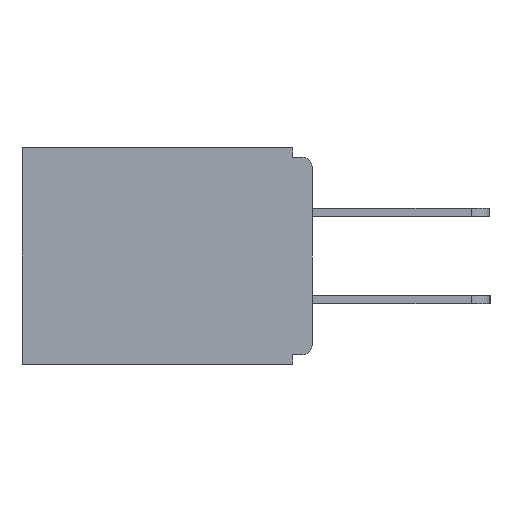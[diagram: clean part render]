
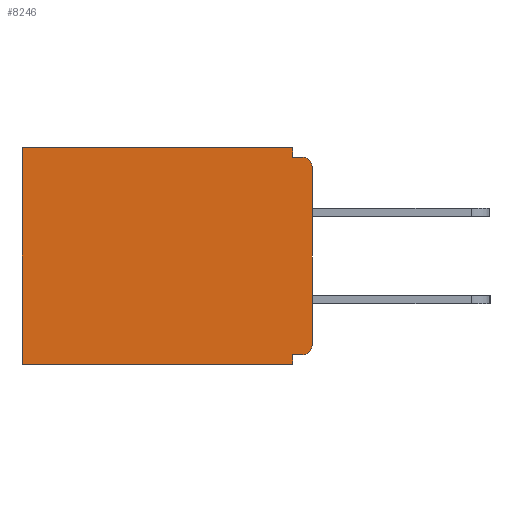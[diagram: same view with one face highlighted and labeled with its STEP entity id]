
A CAD part, left-side view. The second image highlights one B-rep face of the part: STEP entity #8246.
In plain terms, the highlighted planar face has unit normal (-1, 0, 0).
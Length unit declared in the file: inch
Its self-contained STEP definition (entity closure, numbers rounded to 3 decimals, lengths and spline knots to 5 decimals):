
#279 = VECTOR ( 'NONE', #2472, 39.37008 ) ;
#393 = VERTEX_POINT ( 'NONE', #2264 ) ;
#464 = CARTESIAN_POINT ( 'NONE',  ( 0.298, 0.031, -0.343 ) ) ;
#641 = DIRECTION ( 'NONE',  ( 0., 0., -1. ) ) ;
#651 = VERTEX_POINT ( 'NONE', #9952 ) ;
#726 = CARTESIAN_POINT ( 'NONE',  ( 0.298, 0., -0.328 ) ) ;
#794 = VERTEX_POINT ( 'NONE', #1042 ) ;
#1023 = LINE ( 'NONE', #1799, #2054 ) ;
#1042 = CARTESIAN_POINT ( 'NONE',  ( 0.298, 0.015, -0.328 ) ) ;
#1272 = VECTOR ( 'NONE', #8015, 39.37008 ) ;
#1454 = ORIENTED_EDGE ( 'NONE', *, *, #10902, .T. ) ;
#1741 = EDGE_CURVE ( 'NONE', #5971, #651, #8918, .T. ) ;
#1799 = CARTESIAN_POINT ( 'NONE',  ( 0.298, 0., -0.015 ) ) ;
#1800 = CIRCLE ( 'NONE', #10659, 0.015 ) ;
#1918 = ORIENTED_EDGE ( 'NONE', *, *, #3690, .F. ) ;
#2054 = VECTOR ( 'NONE', #12324, 39.37008 ) ;
#2264 = CARTESIAN_POINT ( 'NONE',  ( 0.298, 0.031, -0.015 ) ) ;
#2284 = LINE ( 'NONE', #4852, #12710 ) ;
#2448 = ORIENTED_EDGE ( 'NONE', *, *, #1741, .F. ) ;
#2472 = DIRECTION ( 'NONE',  ( 0., 0., -1. ) ) ;
#2620 = DIRECTION ( 'NONE',  ( -1., 0., 0. ) ) ;
#2828 = PLANE ( 'NONE',  #9819 ) ;
#3073 = VERTEX_POINT ( 'NONE', #3574 ) ;
#3208 = ORIENTED_EDGE ( 'NONE', *, *, #4768, .T. ) ;
#3418 = ORIENTED_EDGE ( 'NONE', *, *, #12832, .T. ) ;
#3472 = CARTESIAN_POINT ( 'NONE',  ( 0.298, 0., 0. ) ) ;
#3574 = CARTESIAN_POINT ( 'NONE',  ( 0.298, 0.031, 0. ) ) ;
#3594 = FACE_OUTER_BOUND ( 'NONE', #8398, .T. ) ;
#3690 = EDGE_CURVE ( 'NONE', #794, #4728, #9856, .T. ) ;
#3745 = VERTEX_POINT ( 'NONE', #13496 ) ;
#3828 = CARTESIAN_POINT ( 'NONE',  ( 0.298, 0.031, -0.328 ) ) ;
#4167 = DIRECTION ( 'NONE',  ( -1., 0., 0. ) ) ;
#4298 = CARTESIAN_POINT ( 'NONE',  ( 0.298, 0.015, -0.313 ) ) ;
#4319 = VECTOR ( 'NONE', #5963, 39.37008 ) ;
#4413 = DIRECTION ( 'NONE',  ( 0., 0., -1. ) ) ;
#4554 = DIRECTION ( 'NONE',  ( 0., 1., 0. ) ) ;
#4728 = VERTEX_POINT ( 'NONE', #3828 ) ;
#4768 = EDGE_CURVE ( 'NONE', #5971, #13236, #5404, .T. ) ;
#4852 = CARTESIAN_POINT ( 'NONE',  ( 0.298, 0., -0.343 ) ) ;
#4991 = LINE ( 'NONE', #464, #279 ) ;
#5404 = CIRCLE ( 'NONE', #7848, 0.015 ) ;
#5413 = EDGE_CURVE ( 'NONE', #794, #651, #1800, .T. ) ;
#5963 = DIRECTION ( 'NONE',  ( 0., 1., 0. ) ) ;
#5968 = EDGE_CURVE ( 'NONE', #8989, #3745, #2284, .T. ) ;
#5971 = VERTEX_POINT ( 'NONE', #11239 ) ;
#6232 = VECTOR ( 'NONE', #4554, 39.37008 ) ;
#6331 = VECTOR ( 'NONE', #9665, 39.37008 ) ;
#6560 = ORIENTED_EDGE ( 'NONE', *, *, #7855, .F. ) ;
#6593 = VECTOR ( 'NONE', #4413, 39.37008 ) ;
#6707 = LINE ( 'NONE', #3472, #6232 ) ;
#6927 = CARTESIAN_POINT ( 'NONE',  ( 0.298, 0., 0. ) ) ;
#7169 = CARTESIAN_POINT ( 'NONE',  ( 0.298, 0.031, -0.343 ) ) ;
#7713 = VERTEX_POINT ( 'NONE', #8289 ) ;
#7799 = LINE ( 'NONE', #11717, #6331 ) ;
#7848 = AXIS2_PLACEMENT_3D ( 'NONE', #11018, #2620, #10045 ) ;
#7855 = EDGE_CURVE ( 'NONE', #3073, #393, #7799, .T. ) ;
#7961 = EDGE_CURVE ( 'NONE', #393, #13236, #1023, .T. ) ;
#8015 = DIRECTION ( 'NONE',  ( 0., 0., -1. ) ) ;
#8246 = ADVANCED_FACE ( 'NONE', ( #3594 ), #2828, .F. ) ;
#8289 = CARTESIAN_POINT ( 'NONE',  ( 0.298, 0.46, 0. ) ) ;
#8398 = EDGE_LOOP ( 'NONE', ( #3208, #10143, #6560, #3418, #1454, #13165, #8598, #1918, #12893, #2448 ) ) ;
#8598 = ORIENTED_EDGE ( 'NONE', *, *, #9366, .F. ) ;
#8918 = LINE ( 'NONE', #6927, #1272 ) ;
#8989 = VERTEX_POINT ( 'NONE', #7169 ) ;
#9366 = EDGE_CURVE ( 'NONE', #4728, #8989, #4991, .T. ) ;
#9665 = DIRECTION ( 'NONE',  ( 0., 0., -1. ) ) ;
#9819 = AXIS2_PLACEMENT_3D ( 'NONE', #13175, #10062, #641 ) ;
#9856 = LINE ( 'NONE', #726, #4319 ) ;
#9952 = CARTESIAN_POINT ( 'NONE',  ( 0.298, 0., -0.313 ) ) ;
#10045 = DIRECTION ( 'NONE',  ( 0., 0., -1. ) ) ;
#10062 = DIRECTION ( 'NONE',  ( 1., 0., 0. ) ) ;
#10081 = DIRECTION ( 'NONE',  ( 0., 1., 0. ) ) ;
#10143 = ORIENTED_EDGE ( 'NONE', *, *, #7961, .F. ) ;
#10659 = AXIS2_PLACEMENT_3D ( 'NONE', #4298, #4167, #13509 ) ;
#10706 = CARTESIAN_POINT ( 'NONE',  ( 0.298, 0.46, 0. ) ) ;
#10902 = EDGE_CURVE ( 'NONE', #7713, #3745, #12144, .T. ) ;
#11018 = CARTESIAN_POINT ( 'NONE',  ( 0.298, 0.015, -0.03 ) ) ;
#11239 = CARTESIAN_POINT ( 'NONE',  ( 0.298, 0., -0.03 ) ) ;
#11717 = CARTESIAN_POINT ( 'NONE',  ( 0.298, 0.031, -0.343 ) ) ;
#12144 = LINE ( 'NONE', #10706, #6593 ) ;
#12324 = DIRECTION ( 'NONE',  ( 0., -1., 0. ) ) ;
#12637 = CARTESIAN_POINT ( 'NONE',  ( 0.298, 0.015, -0.015 ) ) ;
#12710 = VECTOR ( 'NONE', #10081, 39.37008 ) ;
#12832 = EDGE_CURVE ( 'NONE', #3073, #7713, #6707, .T. ) ;
#12893 = ORIENTED_EDGE ( 'NONE', *, *, #5413, .T. ) ;
#13165 = ORIENTED_EDGE ( 'NONE', *, *, #5968, .F. ) ;
#13175 = CARTESIAN_POINT ( 'NONE',  ( 0.298, 0., 0. ) ) ;
#13236 = VERTEX_POINT ( 'NONE', #12637 ) ;
#13496 = CARTESIAN_POINT ( 'NONE',  ( 0.298, 0.46, -0.343 ) ) ;
#13509 = DIRECTION ( 'NONE',  ( 0., 0., -1. ) ) ;
